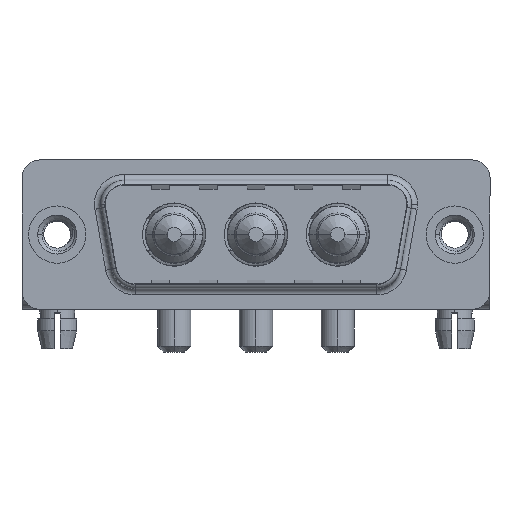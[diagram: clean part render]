
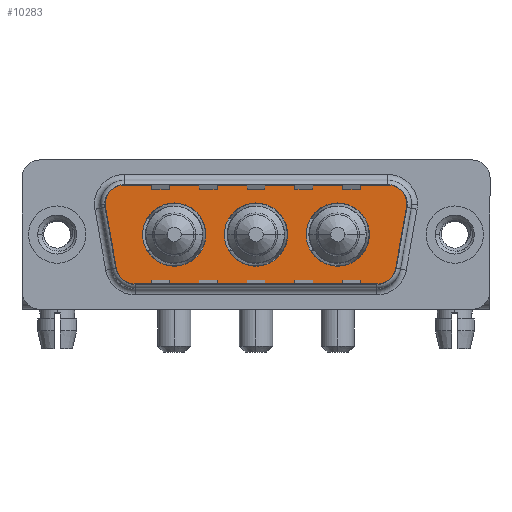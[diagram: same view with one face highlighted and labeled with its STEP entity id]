
A CAD part, top view. The second image highlights one B-rep face of the part: STEP entity #10283.
In plain terms, the highlighted planar face has unit normal (0, 0, 1).
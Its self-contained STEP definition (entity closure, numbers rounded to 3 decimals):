
#34 = DIRECTION ( 'NONE',  ( -1., 0., 0. ) ) ;
#174 = PLANE ( 'NONE',  #5373 ) ;
#188 = CIRCLE ( 'NONE', #2160, 2.65 ) ;
#252 = FACE_BOUND ( 'NONE', #10401, .T. ) ;
#433 = ORIENTED_EDGE ( 'NONE', *, *, #15078, .T. ) ;
#486 = VERTEX_POINT ( 'NONE', #9052 ) ;
#512 = CIRCLE ( 'NONE', #8480, 2.65 ) ;
#813 = AXIS2_PLACEMENT_3D ( 'NONE', #3202, #6735, #2895 ) ;
#1059 = ORIENTED_EDGE ( 'NONE', *, *, #11792, .F. ) ;
#1070 = VERTEX_POINT ( 'NONE', #9515 ) ;
#1280 = ORIENTED_EDGE ( 'NONE', *, *, #10172, .T. ) ;
#1574 = CARTESIAN_POINT ( 'NONE',  ( 26.866, -4.9, 0. ) ) ;
#1679 = CARTESIAN_POINT ( 'NONE',  ( 5.411, 2.9, 0. ) ) ;
#1837 = DIRECTION ( 'NONE',  ( 1., 0., 0. ) ) ;
#1904 = EDGE_CURVE ( 'NONE', #4999, #3623, #4182, .T. ) ;
#1929 = EDGE_CURVE ( 'NONE', #5446, #2708, #3181, .T. ) ;
#2050 = CARTESIAN_POINT ( 'NONE',  ( 5.411, 4.9, 0. ) ) ;
#2098 = VECTOR ( 'NONE', #4666, 1000. ) ;
#2160 = AXIS2_PLACEMENT_3D ( 'NONE', #4203, #6408, #14795 ) ;
#2322 = CARTESIAN_POINT ( 'NONE',  ( 6.434, -4.9, 0. ) ) ;
#2330 = ORIENTED_EDGE ( 'NONE', *, *, #1929, .T. ) ;
#2352 = DIRECTION ( 'NONE',  ( -1., 0., 0. ) ) ;
#2447 = CARTESIAN_POINT ( 'NONE',  ( 26.866, -2.9, 0. ) ) ;
#2527 = DIRECTION ( 'NONE',  ( 0., 0., 1. ) ) ;
#2606 = VECTOR ( 'NONE', #3890, 1000. ) ;
#2609 = ORIENTED_EDGE ( 'NONE', *, *, #1904, .T. ) ;
#2670 = CIRCLE ( 'NONE', #11421, 2. ) ;
#2708 = VERTEX_POINT ( 'NONE', #11702 ) ;
#2752 = CIRCLE ( 'NONE', #13258, 2.65 ) ;
#2765 = CARTESIAN_POINT ( 'NONE',  ( 14., 0., 0. ) ) ;
#2792 = EDGE_CURVE ( 'NONE', #4040, #486, #2670, .T. ) ;
#2855 = DIRECTION ( 'NONE',  ( 1., 0., 0. ) ) ;
#2895 = DIRECTION ( 'NONE',  ( 1., 0., 0. ) ) ;
#2930 = CARTESIAN_POINT ( 'NONE',  ( 6.434, -4.9, 0. ) ) ;
#3017 = DIRECTION ( 'NONE',  ( 0., 0., 1. ) ) ;
#3103 = VERTEX_POINT ( 'NONE', #5504 ) ;
#3181 = CIRCLE ( 'NONE', #4680, 2. ) ;
#3202 = CARTESIAN_POINT ( 'NONE',  ( 16.65, 0., 0. ) ) ;
#3269 = ORIENTED_EDGE ( 'NONE', *, *, #7471, .T. ) ;
#3476 = LINE ( 'NONE', #9212, #14344 ) ;
#3566 = CIRCLE ( 'NONE', #14334, 2.65 ) ;
#3614 = DIRECTION ( 'NONE',  ( 1., 0., 0. ) ) ;
#3617 = CIRCLE ( 'NONE', #5889, 2. ) ;
#3623 = VERTEX_POINT ( 'NONE', #2930 ) ;
#3670 = CARTESIAN_POINT ( 'NONE',  ( 27.889, 2.9, 0. ) ) ;
#3798 = ORIENTED_EDGE ( 'NONE', *, *, #11608, .F. ) ;
#3805 = DIRECTION ( 'NONE',  ( 1., 0., 0. ) ) ;
#3890 = DIRECTION ( 'NONE',  ( 0.174, -0.985, 0. ) ) ;
#4029 = DIRECTION ( 'NONE',  ( 0., 0., 1. ) ) ;
#4040 = VERTEX_POINT ( 'NONE', #1574 ) ;
#4182 = CIRCLE ( 'NONE', #15207, 2. ) ;
#4203 = CARTESIAN_POINT ( 'NONE',  ( 23.5, 0., 0. ) ) ;
#4204 = EDGE_LOOP ( 'NONE', ( #7400, #10251 ) ) ;
#4552 = CARTESIAN_POINT ( 'NONE',  ( 27.889, 4.9, 0. ) ) ;
#4666 = DIRECTION ( 'NONE',  ( 1., 0., 0. ) ) ;
#4680 = AXIS2_PLACEMENT_3D ( 'NONE', #3670, #10495, #7055 ) ;
#4701 = DIRECTION ( 'NONE',  ( 0., 0., 1. ) ) ;
#4917 = CARTESIAN_POINT ( 'NONE',  ( 26.866, -2.9, 0. ) ) ;
#4989 = FACE_BOUND ( 'NONE', #4204, .T. ) ;
#4999 = VERTEX_POINT ( 'NONE', #7832 ) ;
#5373 = AXIS2_PLACEMENT_3D ( 'NONE', #4917, #14561, #3805 ) ;
#5446 = VERTEX_POINT ( 'NONE', #6244 ) ;
#5504 = CARTESIAN_POINT ( 'NONE',  ( 12.45, 0., 0. ) ) ;
#5551 = CARTESIAN_POINT ( 'NONE',  ( 23.5, 0., 0. ) ) ;
#5732 = EDGE_CURVE ( 'NONE', #3103, #11353, #2752, .T. ) ;
#5759 = LINE ( 'NONE', #7002, #10838 ) ;
#5889 = AXIS2_PLACEMENT_3D ( 'NONE', #1679, #3017, #13599 ) ;
#6032 = CARTESIAN_POINT ( 'NONE',  ( 27.889, 2.9, 0. ) ) ;
#6226 = VERTEX_POINT ( 'NONE', #2765 ) ;
#6244 = CARTESIAN_POINT ( 'NONE',  ( 29.859, 2.553, 0. ) ) ;
#6408 = DIRECTION ( 'NONE',  ( 0., 0., 1. ) ) ;
#6467 = CARTESIAN_POINT ( 'NONE',  ( 16.65, 0., 0. ) ) ;
#6529 = VERTEX_POINT ( 'NONE', #7200 ) ;
#6728 = DIRECTION ( 'NONE',  ( 0., 0., 1. ) ) ;
#6735 = DIRECTION ( 'NONE',  ( 0., 0., 1. ) ) ;
#6843 = AXIS2_PLACEMENT_3D ( 'NONE', #6467, #9053, #1837 ) ;
#7002 = CARTESIAN_POINT ( 'NONE',  ( 29.859, 2.553, 0. ) ) ;
#7055 = DIRECTION ( 'NONE',  ( -1., 0., 0. ) ) ;
#7180 = CARTESIAN_POINT ( 'NONE',  ( 19.3, 0., 0. ) ) ;
#7200 = CARTESIAN_POINT ( 'NONE',  ( 26.15, 0., 0. ) ) ;
#7400 = ORIENTED_EDGE ( 'NONE', *, *, #5732, .F. ) ;
#7471 = EDGE_CURVE ( 'NONE', #2708, #12205, #15309, .T. ) ;
#7641 = CARTESIAN_POINT ( 'NONE',  ( 9.8, 0., 0. ) ) ;
#7832 = CARTESIAN_POINT ( 'NONE',  ( 4.464, -3.247, 0. ) ) ;
#7840 = EDGE_CURVE ( 'NONE', #13237, #6226, #14304, .T. ) ;
#8218 = LINE ( 'NONE', #8759, #2606 ) ;
#8305 = AXIS2_PLACEMENT_3D ( 'NONE', #6032, #10578, #2352 ) ;
#8363 = ORIENTED_EDGE ( 'NONE', *, *, #14647, .F. ) ;
#8480 = AXIS2_PLACEMENT_3D ( 'NONE', #5551, #14230, #13061 ) ;
#8759 = CARTESIAN_POINT ( 'NONE',  ( 3.441, 2.553, 0. ) ) ;
#9052 = CARTESIAN_POINT ( 'NONE',  ( 28.836, -3.247, 0. ) ) ;
#9053 = DIRECTION ( 'NONE',  ( 0., 0., 1. ) ) ;
#9212 = CARTESIAN_POINT ( 'NONE',  ( 5.411, 4.9, 0. ) ) ;
#9515 = CARTESIAN_POINT ( 'NONE',  ( 3.441, 2.553, 0. ) ) ;
#9571 = EDGE_CURVE ( 'NONE', #486, #5446, #5759, .T. ) ;
#9767 = EDGE_LOOP ( 'NONE', ( #11737, #14660, #2330, #3269, #14572, #10125, #1280, #2609, #433 ) ) ;
#9775 = FACE_OUTER_BOUND ( 'NONE', #9767, .T. ) ;
#10125 = ORIENTED_EDGE ( 'NONE', *, *, #13412, .T. ) ;
#10172 = EDGE_CURVE ( 'NONE', #1070, #4999, #8218, .T. ) ;
#10245 = DIRECTION ( 'NONE',  ( 1., 0., 0. ) ) ;
#10251 = ORIENTED_EDGE ( 'NONE', *, *, #14248, .F. ) ;
#10283 = ADVANCED_FACE ( 'NONE', ( #252, #14637, #4989, #9775 ), #174, .T. ) ;
#10342 = CIRCLE ( 'NONE', #6843, 2.65 ) ;
#10401 = EDGE_LOOP ( 'NONE', ( #15037, #8363 ) ) ;
#10495 = DIRECTION ( 'NONE',  ( 0., 0., 1. ) ) ;
#10521 = DIRECTION ( 'NONE',  ( 0.174, 0.985, 0. ) ) ;
#10578 = DIRECTION ( 'NONE',  ( 0., 0., 1. ) ) ;
#10615 = VERTEX_POINT ( 'NONE', #2050 ) ;
#10838 = VECTOR ( 'NONE', #10521, 1000. ) ;
#11353 = VERTEX_POINT ( 'NONE', #12277 ) ;
#11421 = AXIS2_PLACEMENT_3D ( 'NONE', #2447, #2527, #3614 ) ;
#11438 = EDGE_LOOP ( 'NONE', ( #3798, #1059 ) ) ;
#11608 = EDGE_CURVE ( 'NONE', #6529, #12375, #188, .T. ) ;
#11702 = CARTESIAN_POINT ( 'NONE',  ( 29.889, 2.9, 0. ) ) ;
#11737 = ORIENTED_EDGE ( 'NONE', *, *, #2792, .T. ) ;
#11792 = EDGE_CURVE ( 'NONE', #12375, #6529, #512, .T. ) ;
#11802 = LINE ( 'NONE', #2322, #2098 ) ;
#12205 = VERTEX_POINT ( 'NONE', #4552 ) ;
#12277 = CARTESIAN_POINT ( 'NONE',  ( 7.15, 0., 0. ) ) ;
#12375 = VERTEX_POINT ( 'NONE', #14663 ) ;
#13014 = CARTESIAN_POINT ( 'NONE',  ( 6.434, -2.9, 0. ) ) ;
#13061 = DIRECTION ( 'NONE',  ( 1., 0., 0. ) ) ;
#13237 = VERTEX_POINT ( 'NONE', #7180 ) ;
#13258 = AXIS2_PLACEMENT_3D ( 'NONE', #7641, #4029, #2855 ) ;
#13412 = EDGE_CURVE ( 'NONE', #10615, #1070, #3617, .T. ) ;
#13599 = DIRECTION ( 'NONE',  ( 1., 0., 0. ) ) ;
#13706 = CARTESIAN_POINT ( 'NONE',  ( 9.8, 0., 0. ) ) ;
#14230 = DIRECTION ( 'NONE',  ( 0., 0., 1. ) ) ;
#14248 = EDGE_CURVE ( 'NONE', #11353, #3103, #3566, .T. ) ;
#14304 = CIRCLE ( 'NONE', #813, 2.65 ) ;
#14334 = AXIS2_PLACEMENT_3D ( 'NONE', #13706, #6728, #10245 ) ;
#14344 = VECTOR ( 'NONE', #15166, 1000. ) ;
#14561 = DIRECTION ( 'NONE',  ( 0., 0., 1. ) ) ;
#14572 = ORIENTED_EDGE ( 'NONE', *, *, #14767, .T. ) ;
#14637 = FACE_BOUND ( 'NONE', #11438, .T. ) ;
#14647 = EDGE_CURVE ( 'NONE', #6226, #13237, #10342, .T. ) ;
#14660 = ORIENTED_EDGE ( 'NONE', *, *, #9571, .T. ) ;
#14663 = CARTESIAN_POINT ( 'NONE',  ( 20.85, 0., 0. ) ) ;
#14767 = EDGE_CURVE ( 'NONE', #12205, #10615, #3476, .T. ) ;
#14795 = DIRECTION ( 'NONE',  ( 1., 0., 0. ) ) ;
#15037 = ORIENTED_EDGE ( 'NONE', *, *, #7840, .F. ) ;
#15078 = EDGE_CURVE ( 'NONE', #3623, #4040, #11802, .T. ) ;
#15166 = DIRECTION ( 'NONE',  ( -1., 0., 0. ) ) ;
#15207 = AXIS2_PLACEMENT_3D ( 'NONE', #13014, #4701, #34 ) ;
#15309 = CIRCLE ( 'NONE', #8305, 2. ) ;
